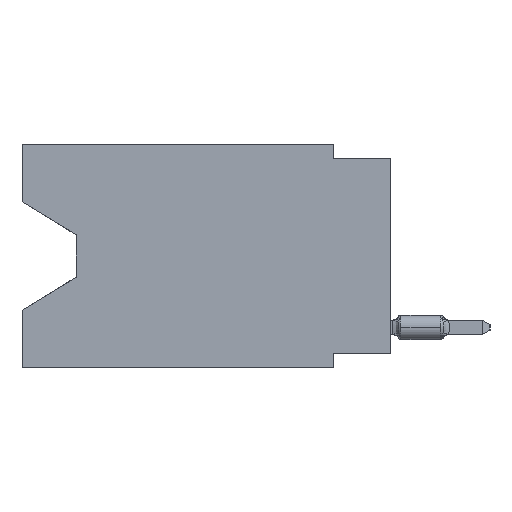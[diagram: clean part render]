
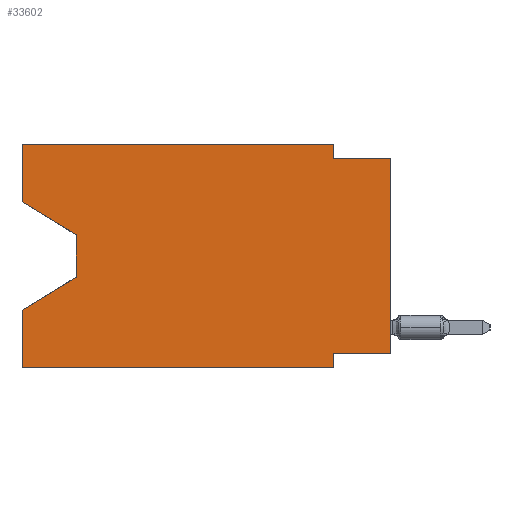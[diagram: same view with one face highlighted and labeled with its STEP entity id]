
A CAD part, left-side view. The second image highlights one B-rep face of the part: STEP entity #33602.
In plain terms, the highlighted planar face has unit normal (-1, 0, 0).
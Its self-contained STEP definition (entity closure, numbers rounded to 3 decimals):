
#204 = CARTESIAN_POINT ( 'NONE',  ( 0., 16.383, 0. ) ) ;
#1683 = VERTEX_POINT ( 'NONE', #47717 ) ;
#3561 = DIRECTION ( 'NONE',  ( 0., 0., -1. ) ) ;
#3602 = EDGE_CURVE ( 'NONE', #42600, #17566, #49592, .T. ) ;
#5328 = VECTOR ( 'NONE', #83908, 1000. ) ;
#7478 = VERTEX_POINT ( 'NONE', #28361 ) ;
#10156 = LINE ( 'NONE', #36063, #54513 ) ;
#10568 = VECTOR ( 'NONE', #62345, 1000. ) ;
#10812 = CARTESIAN_POINT ( 'NONE',  ( 0., 0., 0. ) ) ;
#10899 = EDGE_CURVE ( 'NONE', #50966, #48320, #23509, .T. ) ;
#10920 = CARTESIAN_POINT ( 'NONE',  ( 0., 16.383, -2.546 ) ) ;
#11263 = ORIENTED_EDGE ( 'NONE', *, *, #41855, .F. ) ;
#11920 = CARTESIAN_POINT ( 'NONE',  ( 0., 0., -0.635 ) ) ;
#12306 = EDGE_CURVE ( 'NONE', #29446, #30412, #67769, .T. ) ;
#13342 = ORIENTED_EDGE ( 'NONE', *, *, #28070, .F. ) ;
#14635 = DIRECTION ( 'NONE',  ( 0., 0., 1. ) ) ;
#15379 = CARTESIAN_POINT ( 'NONE',  ( 0., 2.54, 0. ) ) ;
#16187 = ORIENTED_EDGE ( 'NONE', *, *, #53425, .T. ) ;
#16674 = CARTESIAN_POINT ( 'NONE',  ( 0., 16.383, 0. ) ) ;
#16698 = EDGE_LOOP ( 'NONE', ( #63318, #22736, #26706, #80535, #56376, #11263, #13342, #16187, #60801, #18387, #74396, #56199 ) ) ;
#17542 = DIRECTION ( 'NONE',  ( 0., -1., 0. ) ) ;
#17566 = VERTEX_POINT ( 'NONE', #28499 ) ;
#17668 = DIRECTION ( 'NONE',  ( 0., 0., -1. ) ) ;
#18092 = CARTESIAN_POINT ( 'NONE',  ( 0., 2.54, -9.906 ) ) ;
#18387 = ORIENTED_EDGE ( 'NONE', *, *, #51097, .F. ) ;
#19140 = LINE ( 'NONE', #39095, #67021 ) ;
#20409 = DIRECTION ( 'NONE',  ( 0., 1., 0. ) ) ;
#21247 = EDGE_CURVE ( 'NONE', #62449, #7478, #75102, .T. ) ;
#22736 = ORIENTED_EDGE ( 'NONE', *, *, #78914, .T. ) ;
#23509 = LINE ( 'NONE', #43451, #72388 ) ;
#23850 = EDGE_CURVE ( 'NONE', #42600, #29446, #46930, .T. ) ;
#25091 = VECTOR ( 'NONE', #72474, 1000. ) ;
#26706 = ORIENTED_EDGE ( 'NONE', *, *, #48541, .T. ) ;
#27826 = CARTESIAN_POINT ( 'NONE',  ( 0., 16.383, 0. ) ) ;
#28070 = EDGE_CURVE ( 'NONE', #1683, #82050, #79448, .T. ) ;
#28361 = CARTESIAN_POINT ( 'NONE',  ( 0., 2.54, -9.906 ) ) ;
#28376 = DIRECTION ( 'NONE',  ( 0., -1., 0. ) ) ;
#28499 = CARTESIAN_POINT ( 'NONE',  ( 0., 13.97, -4.013 ) ) ;
#28699 = VERTEX_POINT ( 'NONE', #30876 ) ;
#29446 = VERTEX_POINT ( 'NONE', #16674 ) ;
#30412 = VERTEX_POINT ( 'NONE', #15379 ) ;
#30876 = CARTESIAN_POINT ( 'NONE',  ( 0., 13.97, -5.893 ) ) ;
#31687 = LINE ( 'NONE', #18092, #73844 ) ;
#32221 = EDGE_CURVE ( 'NONE', #62449, #39908, #78363, .T. ) ;
#33356 = VECTOR ( 'NONE', #81346, 1000. ) ;
#33602 = ADVANCED_FACE ( 'NONE', ( #41376 ), #34175, .F. ) ;
#34175 = PLANE ( 'NONE',  #63676 ) ;
#36063 = CARTESIAN_POINT ( 'NONE',  ( 0., 13.97, -5.893 ) ) ;
#36231 = VECTOR ( 'NONE', #28376, 1000. ) ;
#36598 = CARTESIAN_POINT ( 'NONE',  ( 0., 2.54, -0.635 ) ) ;
#39095 = CARTESIAN_POINT ( 'NONE',  ( 0., 2.54, 0. ) ) ;
#39908 = VERTEX_POINT ( 'NONE', #42564 ) ;
#41376 = FACE_OUTER_BOUND ( 'NONE', #16698, .T. ) ;
#41600 = VECTOR ( 'NONE', #20409, 1000. ) ;
#41855 = EDGE_CURVE ( 'NONE', #82050, #7478, #31687, .T. ) ;
#42008 = DIRECTION ( 'NONE',  ( 0., 0.855, -0.519 ) ) ;
#42564 = CARTESIAN_POINT ( 'NONE',  ( 0., 16.383, -7.36 ) ) ;
#42600 = VERTEX_POINT ( 'NONE', #54002 ) ;
#43451 = CARTESIAN_POINT ( 'NONE',  ( 0., 0., -0.635 ) ) ;
#46930 = LINE ( 'NONE', #27826, #81038 ) ;
#47717 = CARTESIAN_POINT ( 'NONE',  ( 0., 0., -9.271 ) ) ;
#47808 = VECTOR ( 'NONE', #64791, 1000. ) ;
#48320 = VERTEX_POINT ( 'NONE', #11920 ) ;
#48541 = EDGE_CURVE ( 'NONE', #28699, #39908, #10156, .T. ) ;
#49592 = LINE ( 'NONE', #10920, #10568 ) ;
#49955 = LINE ( 'NONE', #64390, #47808 ) ;
#50966 = VERTEX_POINT ( 'NONE', #36598 ) ;
#51097 = EDGE_CURVE ( 'NONE', #30412, #50966, #19140, .T. ) ;
#52276 = DIRECTION ( 'NONE',  ( 0., 0., -1. ) ) ;
#53425 = EDGE_CURVE ( 'NONE', #1683, #48320, #81784, .T. ) ;
#54002 = CARTESIAN_POINT ( 'NONE',  ( 0., 16.383, -2.546 ) ) ;
#54513 = VECTOR ( 'NONE', #42008, 1000. ) ;
#56199 = ORIENTED_EDGE ( 'NONE', *, *, #23850, .F. ) ;
#56376 = ORIENTED_EDGE ( 'NONE', *, *, #21247, .T. ) ;
#60801 = ORIENTED_EDGE ( 'NONE', *, *, #10899, .F. ) ;
#61791 = CARTESIAN_POINT ( 'NONE',  ( 0., 16.383, 0. ) ) ;
#62345 = DIRECTION ( 'NONE',  ( 0., -0.855, -0.519 ) ) ;
#62449 = VERTEX_POINT ( 'NONE', #75674 ) ;
#63318 = ORIENTED_EDGE ( 'NONE', *, *, #3602, .T. ) ;
#63676 = AXIS2_PLACEMENT_3D ( 'NONE', #61791, #67305, #3561 ) ;
#64390 = CARTESIAN_POINT ( 'NONE',  ( 0., 13.97, -4.013 ) ) ;
#64791 = DIRECTION ( 'NONE',  ( 0., 0., -1. ) ) ;
#66291 = CARTESIAN_POINT ( 'NONE',  ( 0., 0., -9.271 ) ) ;
#67021 = VECTOR ( 'NONE', #52276, 1000. ) ;
#67305 = DIRECTION ( 'NONE',  ( 1., 0., 0. ) ) ;
#67769 = LINE ( 'NONE', #74135, #25091 ) ;
#72388 = VECTOR ( 'NONE', #17542, 1000. ) ;
#72474 = DIRECTION ( 'NONE',  ( 0., -1., 0. ) ) ;
#73844 = VECTOR ( 'NONE', #17668, 1000. ) ;
#74135 = CARTESIAN_POINT ( 'NONE',  ( 0., 16.383, 0. ) ) ;
#74396 = ORIENTED_EDGE ( 'NONE', *, *, #12306, .F. ) ;
#74661 = CARTESIAN_POINT ( 'NONE',  ( 0., 16.383, -9.906 ) ) ;
#75102 = LINE ( 'NONE', #74661, #36231 ) ;
#75674 = CARTESIAN_POINT ( 'NONE',  ( 0., 16.383, -9.906 ) ) ;
#76549 = CARTESIAN_POINT ( 'NONE',  ( 0., 2.54, -9.271 ) ) ;
#78363 = LINE ( 'NONE', #204, #5328 ) ;
#78914 = EDGE_CURVE ( 'NONE', #17566, #28699, #49955, .T. ) ;
#79448 = LINE ( 'NONE', #66291, #41600 ) ;
#80535 = ORIENTED_EDGE ( 'NONE', *, *, #32221, .F. ) ;
#81038 = VECTOR ( 'NONE', #14635, 1000. ) ;
#81346 = DIRECTION ( 'NONE',  ( 0., 0., 1. ) ) ;
#81784 = LINE ( 'NONE', #10812, #33356 ) ;
#82050 = VERTEX_POINT ( 'NONE', #76549 ) ;
#83908 = DIRECTION ( 'NONE',  ( 0., 0., 1. ) ) ;
